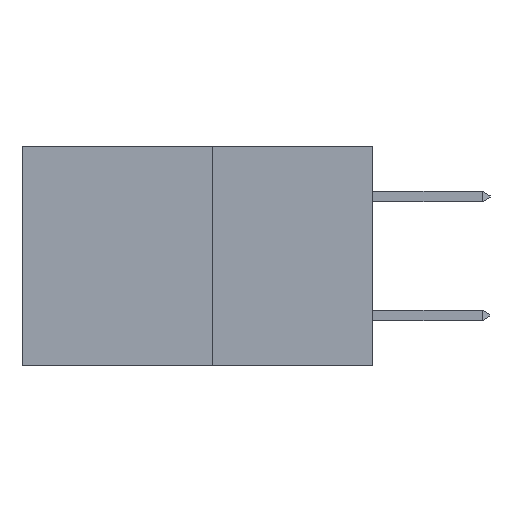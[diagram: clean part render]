
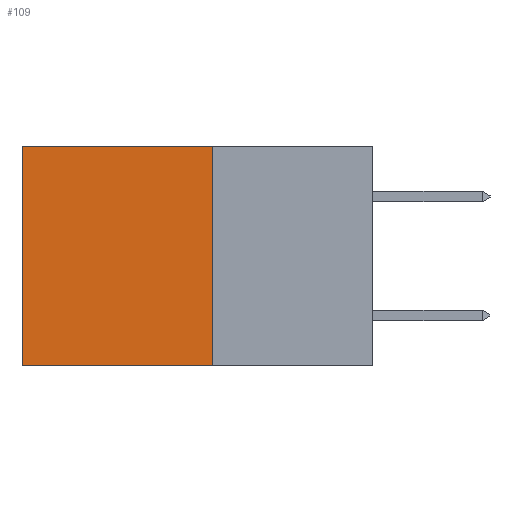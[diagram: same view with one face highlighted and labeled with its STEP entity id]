
A CAD part, left-side view. The second image highlights one B-rep face of the part: STEP entity #109.
In plain terms, the highlighted planar face has unit normal (-1, 0, 0).
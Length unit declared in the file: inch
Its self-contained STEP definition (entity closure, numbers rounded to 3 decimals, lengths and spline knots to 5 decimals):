
#109 = ADVANCED_FACE ( 'NONE', ( #16874 ), #7080, .F. ) ;
#1569 = EDGE_CURVE ( 'NONE', #6397, #14325, #14776, .T. ) ;
#1633 = LINE ( 'NONE', #12196, #12198 ) ;
#1981 = LINE ( 'NONE', #7736, #15705 ) ;
#2111 = CARTESIAN_POINT ( 'NONE',  ( 0.277, 0.59, 0. ) ) ;
#3253 = ORIENTED_EDGE ( 'NONE', *, *, #1569, .T. ) ;
#3374 = DIRECTION ( 'NONE',  ( 0., 0., -1. ) ) ;
#4140 = VECTOR ( 'NONE', #3374, 39.37008 ) ;
#4183 = ORIENTED_EDGE ( 'NONE', *, *, #14821, .T. ) ;
#4269 = DIRECTION ( 'NONE',  ( 0., 0., -1. ) ) ;
#4777 = ORIENTED_EDGE ( 'NONE', *, *, #10659, .F. ) ;
#4904 = ORIENTED_EDGE ( 'NONE', *, *, #10673, .F. ) ;
#6068 = CARTESIAN_POINT ( 'NONE',  ( 0.277, 0.27, -0.37 ) ) ;
#6360 = AXIS2_PLACEMENT_3D ( 'NONE', #6068, #9165, #13587 ) ;
#6397 = VERTEX_POINT ( 'NONE', #2111 ) ;
#6585 = CARTESIAN_POINT ( 'NONE',  ( 0.277, 0.27, 0. ) ) ;
#6657 = CARTESIAN_POINT ( 'NONE',  ( 0.277, 0.59, -0.37 ) ) ;
#7080 = PLANE ( 'NONE',  #6360 ) ;
#7736 = CARTESIAN_POINT ( 'NONE',  ( 0.277, 0.27, 0. ) ) ;
#9165 = DIRECTION ( 'NONE',  ( 1., 0., 0. ) ) ;
#9433 = CARTESIAN_POINT ( 'NONE',  ( 0.277, 0.27, -0.37 ) ) ;
#10596 = CARTESIAN_POINT ( 'NONE',  ( 0.277, 0.27, -0.37 ) ) ;
#10659 = EDGE_CURVE ( 'NONE', #16092, #11971, #15365, .T. ) ;
#10673 = EDGE_CURVE ( 'NONE', #11971, #14325, #1633, .T. ) ;
#11218 = EDGE_LOOP ( 'NONE', ( #3253, #4904, #4777, #4183 ) ) ;
#11751 = VECTOR ( 'NONE', #4269, 39.37008 ) ;
#11801 = DIRECTION ( 'NONE',  ( 0., 1., 0. ) ) ;
#11971 = VERTEX_POINT ( 'NONE', #10596 ) ;
#12190 = CARTESIAN_POINT ( 'NONE',  ( 0.277, 0.59, -0.37 ) ) ;
#12196 = CARTESIAN_POINT ( 'NONE',  ( 0.277, 0.27, -0.37 ) ) ;
#12198 = VECTOR ( 'NONE', #13554, 39.37008 ) ;
#13554 = DIRECTION ( 'NONE',  ( 0., 1., 0. ) ) ;
#13587 = DIRECTION ( 'NONE',  ( 0., 0., -1. ) ) ;
#14325 = VERTEX_POINT ( 'NONE', #12190 ) ;
#14776 = LINE ( 'NONE', #6657, #4140 ) ;
#14821 = EDGE_CURVE ( 'NONE', #16092, #6397, #1981, .T. ) ;
#15365 = LINE ( 'NONE', #9433, #11751 ) ;
#15705 = VECTOR ( 'NONE', #11801, 39.37008 ) ;
#16092 = VERTEX_POINT ( 'NONE', #6585 ) ;
#16874 = FACE_OUTER_BOUND ( 'NONE', #11218, .T. ) ;
